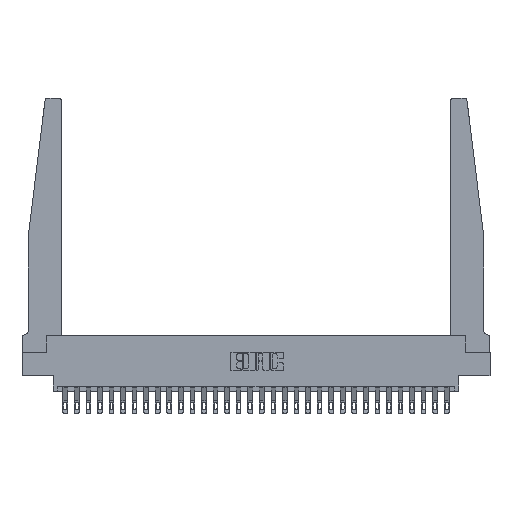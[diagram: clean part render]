
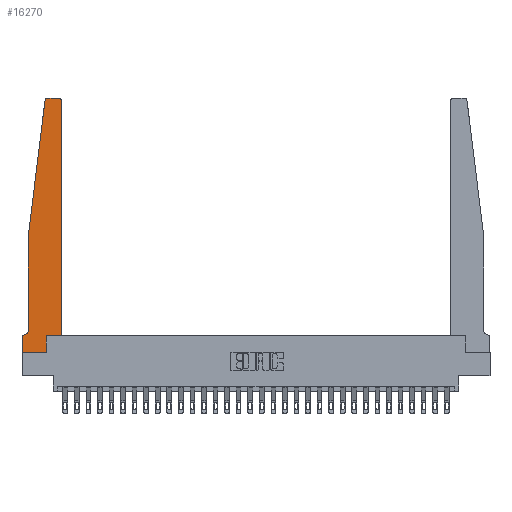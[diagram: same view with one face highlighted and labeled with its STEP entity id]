
A CAD part, top view. The second image highlights one B-rep face of the part: STEP entity #16270.
In plain terms, the highlighted planar face has unit normal (0, 0, 1).
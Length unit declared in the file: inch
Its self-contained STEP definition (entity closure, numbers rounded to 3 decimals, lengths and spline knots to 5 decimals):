
#299 = CIRCLE ( 'NONE', #7780, 0.03 ) ;
#413 = EDGE_CURVE ( 'NONE', #20607, #5645, #24201, .T. ) ;
#455 = CARTESIAN_POINT ( 'NONE',  ( 0.27653, 2.72, 0.37 ) ) ;
#763 = VECTOR ( 'NONE', #4752, 39.37008 ) ;
#870 = VECTOR ( 'NONE', #24512, 39.37008 ) ;
#1498 = EDGE_CURVE ( 'NONE', #11714, #7693, #22210, .T. ) ;
#2058 = VERTEX_POINT ( 'NONE', #5714 ) ;
#2301 = CARTESIAN_POINT ( 'NONE',  ( 0.065, 1.25, 0.37 ) ) ;
#2318 = LINE ( 'NONE', #27242, #23996 ) ;
#2508 = DIRECTION ( 'NONE',  ( -1., 0., 0. ) ) ;
#2852 = CARTESIAN_POINT ( 'NONE',  ( 0.425, 2.72, 0.37 ) ) ;
#3300 = CARTESIAN_POINT ( 'NONE',  ( 0.27653, 2.75, 0.37 ) ) ;
#3544 = DIRECTION ( 'NONE',  ( -1., 0., 0. ) ) ;
#3587 = LINE ( 'NONE', #21480, #870 ) ;
#3978 = CARTESIAN_POINT ( 'NONE',  ( 0.015, 0.1875, 0.37 ) ) ;
#4191 = DIRECTION ( 'NONE',  ( 1., 0., 0. ) ) ;
#4331 = CARTESIAN_POINT ( 'NONE',  ( 0.425, 0.18, 0.37 ) ) ;
#4481 = EDGE_CURVE ( 'NONE', #9984, #8156, #14773, .T. ) ;
#4670 = EDGE_CURVE ( 'NONE', #5645, #10193, #299, .T. ) ;
#4680 = ORIENTED_EDGE ( 'NONE', *, *, #27552, .T. ) ;
#4701 = LINE ( 'NONE', #22574, #17986 ) ;
#4752 = DIRECTION ( 'NONE',  ( 0., 1., 0. ) ) ;
#5405 = DIRECTION ( 'NONE',  ( 0., 0., 1. ) ) ;
#5627 = VECTOR ( 'NONE', #8595, 39.37008 ) ;
#5645 = VERTEX_POINT ( 'NONE', #3300 ) ;
#5714 = CARTESIAN_POINT ( 'NONE',  ( 0.2605, 0., 0.37 ) ) ;
#6031 = CIRCLE ( 'NONE', #27064, 0.03 ) ;
#6441 = VERTEX_POINT ( 'NONE', #17147 ) ;
#7123 = EDGE_CURVE ( 'NONE', #10193, #26299, #20015, .T. ) ;
#7535 = CARTESIAN_POINT ( 'NONE',  ( 0.2605, 0.18, 0.37 ) ) ;
#7693 = VERTEX_POINT ( 'NONE', #10683 ) ;
#7705 = VECTOR ( 'NONE', #3544, 39.37008 ) ;
#7780 = AXIS2_PLACEMENT_3D ( 'NONE', #455, #18632, #20837 ) ;
#8156 = VERTEX_POINT ( 'NONE', #3978 ) ;
#8188 = ORIENTED_EDGE ( 'NONE', *, *, #22951, .T. ) ;
#8299 = EDGE_CURVE ( 'NONE', #16460, #20607, #6031, .T. ) ;
#8595 = DIRECTION ( 'NONE',  ( 0., 1., 0. ) ) ;
#8707 = CARTESIAN_POINT ( 'NONE',  ( 0.065, 1.25, 0.37 ) ) ;
#8802 = CARTESIAN_POINT ( 'NONE',  ( 0.015, 0.2375, 0.37 ) ) ;
#9499 = DIRECTION ( 'NONE',  ( 1., 0., 0. ) ) ;
#9785 = VERTEX_POINT ( 'NONE', #24023 ) ;
#9982 = LINE ( 'NONE', #12038, #17631 ) ;
#9984 = VERTEX_POINT ( 'NONE', #26648 ) ;
#10193 = VERTEX_POINT ( 'NONE', #28537 ) ;
#10358 = EDGE_CURVE ( 'NONE', #7693, #16460, #11488, .T. ) ;
#10683 = CARTESIAN_POINT ( 'NONE',  ( 0.425, 0.18, 0.37 ) ) ;
#10794 = CARTESIAN_POINT ( 'NONE',  ( 0.395, 2.75, 0.37 ) ) ;
#10928 = CARTESIAN_POINT ( 'NONE',  ( 0., 0.1875, 0.37 ) ) ;
#11139 = DIRECTION ( 'NONE',  ( -1., 0., 0. ) ) ;
#11488 = LINE ( 'NONE', #4331, #763 ) ;
#11714 = VERTEX_POINT ( 'NONE', #7535 ) ;
#12038 = CARTESIAN_POINT ( 'NONE',  ( 0.065, 1.25, 0.37 ) ) ;
#12271 = ORIENTED_EDGE ( 'NONE', *, *, #7123, .T. ) ;
#13542 = CARTESIAN_POINT ( 'NONE',  ( 0.2605, 0.18, 0.37 ) ) ;
#14140 = ORIENTED_EDGE ( 'NONE', *, *, #1498, .T. ) ;
#14773 = CIRCLE ( 'NONE', #16667, 0.05 ) ;
#14833 = CARTESIAN_POINT ( 'NONE',  ( 0.25, 2.75, 0.37 ) ) ;
#15299 = ORIENTED_EDGE ( 'NONE', *, *, #413, .T. ) ;
#16242 = EDGE_CURVE ( 'NONE', #2058, #11714, #24273, .T. ) ;
#16270 = ADVANCED_FACE ( 'NONE', ( #26766 ), #28687, .T. ) ;
#16460 = VERTEX_POINT ( 'NONE', #2852 ) ;
#16667 = AXIS2_PLACEMENT_3D ( 'NONE', #8802, #24911, #11139 ) ;
#17147 = CARTESIAN_POINT ( 'NONE',  ( 0., 0.1875, 0.37 ) ) ;
#17484 = VECTOR ( 'NONE', #4191, 39.37008 ) ;
#17631 = VECTOR ( 'NONE', #23468, 39.37008 ) ;
#17665 = DIRECTION ( 'NONE',  ( -0.122, -0.992, 0. ) ) ;
#17688 = DIRECTION ( 'NONE',  ( 1., 0., 0. ) ) ;
#17986 = VECTOR ( 'NONE', #2508, 39.37008 ) ;
#18303 = DIRECTION ( 'NONE',  ( 1., 0., 0. ) ) ;
#18611 = CARTESIAN_POINT ( 'NONE',  ( 0.395, 2.72, 0.37 ) ) ;
#18632 = DIRECTION ( 'NONE',  ( 0., 0., 1. ) ) ;
#18693 = VECTOR ( 'NONE', #17665, 39.37008 ) ;
#19900 = DIRECTION ( 'NONE',  ( 0., 0., 1. ) ) ;
#20015 = LINE ( 'NONE', #8707, #18693 ) ;
#20412 = EDGE_CURVE ( 'NONE', #9785, #2058, #2318, .T. ) ;
#20607 = VERTEX_POINT ( 'NONE', #10794 ) ;
#20837 = DIRECTION ( 'NONE',  ( 1., 0., 0. ) ) ;
#21010 = ORIENTED_EDGE ( 'NONE', *, *, #4481, .T. ) ;
#21480 = CARTESIAN_POINT ( 'NONE',  ( 0., 0., 0.37 ) ) ;
#22210 = LINE ( 'NONE', #28680, #17484 ) ;
#22335 = ORIENTED_EDGE ( 'NONE', *, *, #16242, .T. ) ;
#22574 = CARTESIAN_POINT ( 'NONE',  ( 0.065, 0.1875, 0.37 ) ) ;
#22951 = EDGE_CURVE ( 'NONE', #8156, #6441, #4701, .T. ) ;
#23468 = DIRECTION ( 'NONE',  ( 0., -1., 0. ) ) ;
#23514 = EDGE_LOOP ( 'NONE', ( #15299, #25631, #12271, #4680, #21010, #8188, #23987, #24591, #22335, #14140, #26800, #25377 ) ) ;
#23987 = ORIENTED_EDGE ( 'NONE', *, *, #28850, .T. ) ;
#23996 = VECTOR ( 'NONE', #18303, 39.37008 ) ;
#24023 = CARTESIAN_POINT ( 'NONE',  ( 0., 0., 0.37 ) ) ;
#24201 = LINE ( 'NONE', #14833, #7705 ) ;
#24273 = LINE ( 'NONE', #13542, #5627 ) ;
#24512 = DIRECTION ( 'NONE',  ( 0., -1., 0. ) ) ;
#24591 = ORIENTED_EDGE ( 'NONE', *, *, #20412, .T. ) ;
#24911 = DIRECTION ( 'NONE',  ( 0., 0., -1. ) ) ;
#25377 = ORIENTED_EDGE ( 'NONE', *, *, #8299, .T. ) ;
#25631 = ORIENTED_EDGE ( 'NONE', *, *, #4670, .T. ) ;
#25750 = AXIS2_PLACEMENT_3D ( 'NONE', #10928, #19900, #17688 ) ;
#26299 = VERTEX_POINT ( 'NONE', #2301 ) ;
#26648 = CARTESIAN_POINT ( 'NONE',  ( 0.065, 0.2375, 0.37 ) ) ;
#26766 = FACE_OUTER_BOUND ( 'NONE', #23514, .T. ) ;
#26800 = ORIENTED_EDGE ( 'NONE', *, *, #10358, .T. ) ;
#27064 = AXIS2_PLACEMENT_3D ( 'NONE', #18611, #5405, #9499 ) ;
#27242 = CARTESIAN_POINT ( 'NONE',  ( 0., 0., 0.37 ) ) ;
#27552 = EDGE_CURVE ( 'NONE', #26299, #9984, #9982, .T. ) ;
#28537 = CARTESIAN_POINT ( 'NONE',  ( 0.24675, 2.72367, 0.37 ) ) ;
#28680 = CARTESIAN_POINT ( 'NONE',  ( 0.425, 0.18, 0.37 ) ) ;
#28687 = PLANE ( 'NONE',  #25750 ) ;
#28850 = EDGE_CURVE ( 'NONE', #6441, #9785, #3587, .T. ) ;
